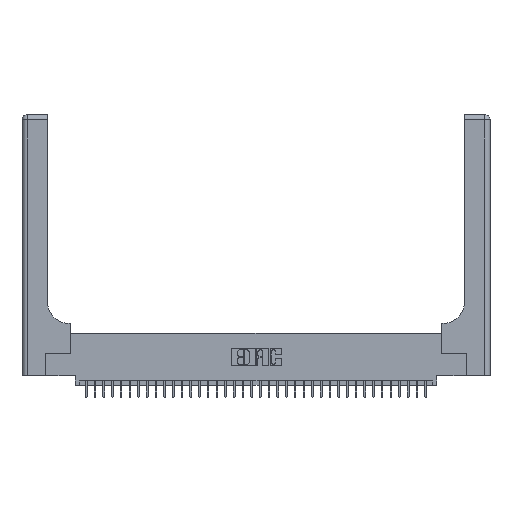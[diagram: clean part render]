
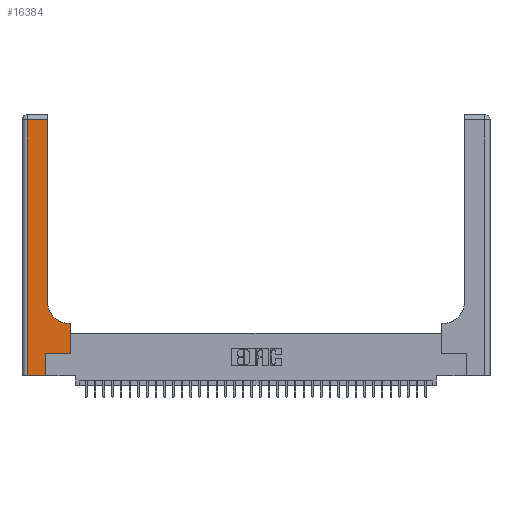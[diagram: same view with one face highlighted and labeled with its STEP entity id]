
A CAD part, top view. The second image highlights one B-rep face of the part: STEP entity #16384.
In plain terms, the highlighted planar face has unit normal (0, 0, 1).
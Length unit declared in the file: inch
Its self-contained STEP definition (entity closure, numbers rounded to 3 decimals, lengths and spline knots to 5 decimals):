
#164 = LINE ( 'NONE', #20749, #15690 ) ;
#509 = EDGE_LOOP ( 'NONE', ( #24005, #11168, #28111, #35810, #34753, #32876, #14414, #22909, #23411 ) ) ;
#866 = EDGE_CURVE ( 'NONE', #19882, #35634, #17664, .T. ) ;
#910 = DIRECTION ( 'NONE',  ( 1., 0., 0. ) ) ;
#1682 = CARTESIAN_POINT ( 'NONE',  ( 0.06, 0., 0.37 ) ) ;
#1750 = CARTESIAN_POINT ( 'NONE',  ( 0., 2.94, 0.37 ) ) ;
#1833 = VECTOR ( 'NONE', #23500, 39.37008 ) ;
#3242 = FACE_OUTER_BOUND ( 'NONE', #509, .T. ) ;
#3421 = PLANE ( 'NONE',  #22838 ) ;
#3448 = CARTESIAN_POINT ( 'NONE',  ( 0.06, 3., 0.37 ) ) ;
#3690 = VECTOR ( 'NONE', #23334, 39.37008 ) ;
#3921 = VERTEX_POINT ( 'NONE', #9368 ) ;
#5983 = DIRECTION ( 'NONE',  ( 0., 0., -1. ) ) ;
#6566 = CARTESIAN_POINT ( 'NONE',  ( 0.5585, 0.6, 0.37 ) ) ;
#8608 = CARTESIAN_POINT ( 'NONE',  ( 0.5415, 0.85, 0.37 ) ) ;
#8631 = CARTESIAN_POINT ( 'NONE',  ( 0.5585, 0.25, 0.37 ) ) ;
#8735 = DIRECTION ( 'NONE',  ( 1., 0., 0. ) ) ;
#9368 = CARTESIAN_POINT ( 'NONE',  ( 0.269, 0.25, 0.37 ) ) ;
#10545 = EDGE_CURVE ( 'NONE', #18963, #27787, #33649, .T. ) ;
#11038 = LINE ( 'NONE', #31417, #3690 ) ;
#11104 = CARTESIAN_POINT ( 'NONE',  ( 0.2915, 3., 0.37 ) ) ;
#11168 = ORIENTED_EDGE ( 'NONE', *, *, #28834, .T. ) ;
#11300 = EDGE_CURVE ( 'NONE', #27787, #23314, #22135, .T. ) ;
#11747 = CARTESIAN_POINT ( 'NONE',  ( 0.2915, 2.94, 0.37 ) ) ;
#13605 = CARTESIAN_POINT ( 'NONE',  ( 0.2915, 0.85, 0.37 ) ) ;
#14414 = ORIENTED_EDGE ( 'NONE', *, *, #10545, .T. ) ;
#14617 = CARTESIAN_POINT ( 'NONE',  ( 0.06, 2.94, 0.37 ) ) ;
#14830 = CARTESIAN_POINT ( 'NONE',  ( 0., 3., 0.37 ) ) ;
#15392 = CARTESIAN_POINT ( 'NONE',  ( 0.5415, 0.6, 0.37 ) ) ;
#15447 = VECTOR ( 'NONE', #18941, 39.37008 ) ;
#15690 = VECTOR ( 'NONE', #910, 39.37008 ) ;
#15909 = EDGE_CURVE ( 'NONE', #35634, #19404, #16995, .T. ) ;
#16384 = ADVANCED_FACE ( 'NONE', ( #3242 ), #3421, .F. ) ;
#16650 = EDGE_CURVE ( 'NONE', #19404, #3921, #11038, .T. ) ;
#16925 = DIRECTION ( 'NONE',  ( 0., 1., 0. ) ) ;
#16995 = LINE ( 'NONE', #23013, #34818 ) ;
#17180 = VECTOR ( 'NONE', #16925, 39.37008 ) ;
#17231 = VECTOR ( 'NONE', #28130, 39.37008 ) ;
#17664 = LINE ( 'NONE', #3448, #1833 ) ;
#17749 = EDGE_CURVE ( 'NONE', #3921, #18963, #164, .T. ) ;
#17809 = DIRECTION ( 'NONE',  ( -1., 0., 0. ) ) ;
#18941 = DIRECTION ( 'NONE',  ( -1., 0., 0. ) ) ;
#18963 = VERTEX_POINT ( 'NONE', #25416 ) ;
#19404 = VERTEX_POINT ( 'NONE', #30806 ) ;
#19882 = VERTEX_POINT ( 'NONE', #14617 ) ;
#20638 = DIRECTION ( 'NONE',  ( 0., 0., -1. ) ) ;
#20749 = CARTESIAN_POINT ( 'NONE',  ( 0.269, 0.25, 0.37 ) ) ;
#20973 = AXIS2_PLACEMENT_3D ( 'NONE', #8608, #5983, #31697 ) ;
#21556 = CIRCLE ( 'NONE', #20973, 0.25 ) ;
#22135 = LINE ( 'NONE', #33636, #15447 ) ;
#22838 = AXIS2_PLACEMENT_3D ( 'NONE', #14830, #20638, #17809 ) ;
#22909 = ORIENTED_EDGE ( 'NONE', *, *, #11300, .T. ) ;
#23013 = CARTESIAN_POINT ( 'NONE',  ( 0., 0., 0.37 ) ) ;
#23314 = VERTEX_POINT ( 'NONE', #15392 ) ;
#23334 = DIRECTION ( 'NONE',  ( 0., 1., 0. ) ) ;
#23411 = ORIENTED_EDGE ( 'NONE', *, *, #31368, .T. ) ;
#23500 = DIRECTION ( 'NONE',  ( 0., -1., 0. ) ) ;
#24005 = ORIENTED_EDGE ( 'NONE', *, *, #25409, .T. ) ;
#25043 = VERTEX_POINT ( 'NONE', #13605 ) ;
#25409 = EDGE_CURVE ( 'NONE', #25043, #29260, #27442, .T. ) ;
#25416 = CARTESIAN_POINT ( 'NONE',  ( 0.5585, 0.25, 0.37 ) ) ;
#27409 = VECTOR ( 'NONE', #31537, 39.37008 ) ;
#27442 = LINE ( 'NONE', #11104, #17180 ) ;
#27787 = VERTEX_POINT ( 'NONE', #6566 ) ;
#28111 = ORIENTED_EDGE ( 'NONE', *, *, #866, .T. ) ;
#28130 = DIRECTION ( 'NONE',  ( -1., 0., 0. ) ) ;
#28834 = EDGE_CURVE ( 'NONE', #29260, #19882, #36057, .T. ) ;
#29260 = VERTEX_POINT ( 'NONE', #11747 ) ;
#30806 = CARTESIAN_POINT ( 'NONE',  ( 0.269, 0., 0.37 ) ) ;
#31368 = EDGE_CURVE ( 'NONE', #23314, #25043, #21556, .T. ) ;
#31417 = CARTESIAN_POINT ( 'NONE',  ( 0.269, 0., 0.37 ) ) ;
#31537 = DIRECTION ( 'NONE',  ( 0., 1., 0. ) ) ;
#31697 = DIRECTION ( 'NONE',  ( 1., 0., 0. ) ) ;
#32876 = ORIENTED_EDGE ( 'NONE', *, *, #17749, .T. ) ;
#33636 = CARTESIAN_POINT ( 'NONE',  ( 0.2915, 0.6, 0.37 ) ) ;
#33649 = LINE ( 'NONE', #8631, #27409 ) ;
#34753 = ORIENTED_EDGE ( 'NONE', *, *, #16650, .T. ) ;
#34818 = VECTOR ( 'NONE', #8735, 39.37008 ) ;
#35634 = VERTEX_POINT ( 'NONE', #1682 ) ;
#35810 = ORIENTED_EDGE ( 'NONE', *, *, #15909, .T. ) ;
#36057 = LINE ( 'NONE', #1750, #17231 ) ;
